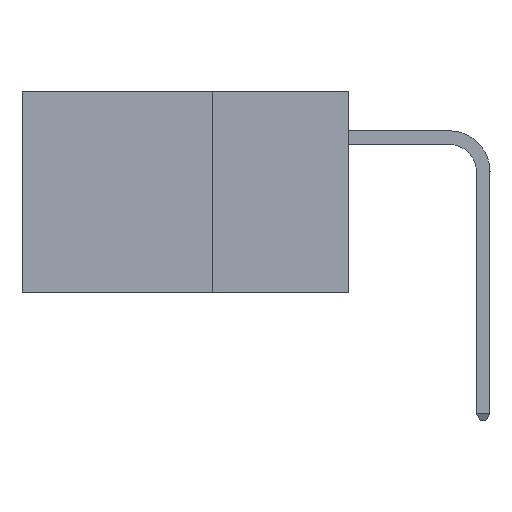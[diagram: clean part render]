
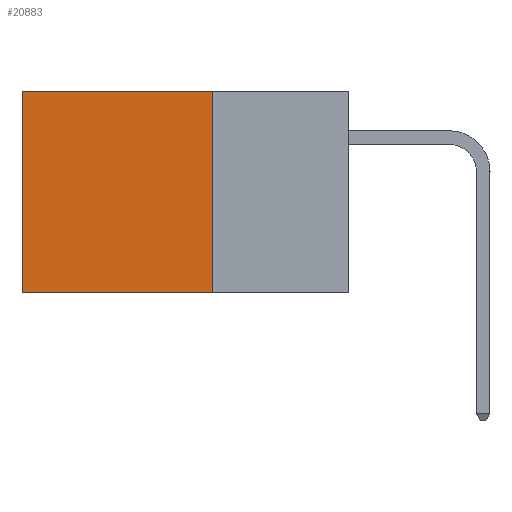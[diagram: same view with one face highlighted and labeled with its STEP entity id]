
A CAD part, left-side view. The second image highlights one B-rep face of the part: STEP entity #20883.
In plain terms, the highlighted planar face has unit normal (-1, 0, 0).
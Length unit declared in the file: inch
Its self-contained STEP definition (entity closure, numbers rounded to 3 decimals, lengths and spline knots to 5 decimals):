
#63 = VERTEX_POINT ( 'NONE', #33755 ) ;
#287 = AXIS2_PLACEMENT_3D ( 'NONE', #7771, #34225, #34348 ) ;
#3208 = DIRECTION ( 'NONE',  ( 0., 0., -1. ) ) ;
#5633 = VECTOR ( 'NONE', #3208, 39.37008 ) ;
#6890 = CARTESIAN_POINT ( 'NONE',  ( 0.2875, 0.6, -0.37 ) ) ;
#7717 = DIRECTION ( 'NONE',  ( 0., 1., 0. ) ) ;
#7771 = CARTESIAN_POINT ( 'NONE',  ( 0.2875, 0.25, 0. ) ) ;
#7819 = CARTESIAN_POINT ( 'NONE',  ( 0.2875, 0.25, 0. ) ) ;
#8473 = CARTESIAN_POINT ( 'NONE',  ( 0.2875, 0.25, 0. ) ) ;
#10849 = LINE ( 'NONE', #27895, #30777 ) ;
#10887 = LINE ( 'NONE', #16512, #30741 ) ;
#11420 = EDGE_CURVE ( 'NONE', #31722, #36531, #13564, .T. ) ;
#12308 = ORIENTED_EDGE ( 'NONE', *, *, #33238, .T. ) ;
#13564 = LINE ( 'NONE', #8473, #5633 ) ;
#16512 = CARTESIAN_POINT ( 'NONE',  ( 0.2875, 0.25, 0. ) ) ;
#18790 = DIRECTION ( 'NONE',  ( 0., 0., -1. ) ) ;
#19181 = CARTESIAN_POINT ( 'NONE',  ( 0.2875, 0.6, 0. ) ) ;
#19352 = VERTEX_POINT ( 'NONE', #6890 ) ;
#20187 = EDGE_CURVE ( 'NONE', #31722, #63, #10887, .T. ) ;
#20883 = ADVANCED_FACE ( 'NONE', ( #33794 ), #21928, .F. ) ;
#21928 = PLANE ( 'NONE',  #287 ) ;
#23615 = LINE ( 'NONE', #19181, #24555 ) ;
#23997 = EDGE_CURVE ( 'NONE', #36531, #19352, #10849, .T. ) ;
#24555 = VECTOR ( 'NONE', #18790, 39.37008 ) ;
#24556 = CARTESIAN_POINT ( 'NONE',  ( 0.2875, 0.25, -0.37 ) ) ;
#25293 = ORIENTED_EDGE ( 'NONE', *, *, #23997, .F. ) ;
#27771 = DIRECTION ( 'NONE',  ( 0., 1., 0. ) ) ;
#27895 = CARTESIAN_POINT ( 'NONE',  ( 0.2875, 0.25, -0.37 ) ) ;
#28845 = ORIENTED_EDGE ( 'NONE', *, *, #11420, .F. ) ;
#28962 = EDGE_LOOP ( 'NONE', ( #12308, #25293, #28845, #31609 ) ) ;
#30741 = VECTOR ( 'NONE', #7717, 39.37008 ) ;
#30777 = VECTOR ( 'NONE', #27771, 39.37008 ) ;
#31609 = ORIENTED_EDGE ( 'NONE', *, *, #20187, .T. ) ;
#31722 = VERTEX_POINT ( 'NONE', #7819 ) ;
#33238 = EDGE_CURVE ( 'NONE', #63, #19352, #23615, .T. ) ;
#33755 = CARTESIAN_POINT ( 'NONE',  ( 0.2875, 0.6, 0. ) ) ;
#33794 = FACE_OUTER_BOUND ( 'NONE', #28962, .T. ) ;
#34225 = DIRECTION ( 'NONE',  ( 1., 0., 0. ) ) ;
#34348 = DIRECTION ( 'NONE',  ( 0., 0., -1. ) ) ;
#36531 = VERTEX_POINT ( 'NONE', #24556 ) ;
